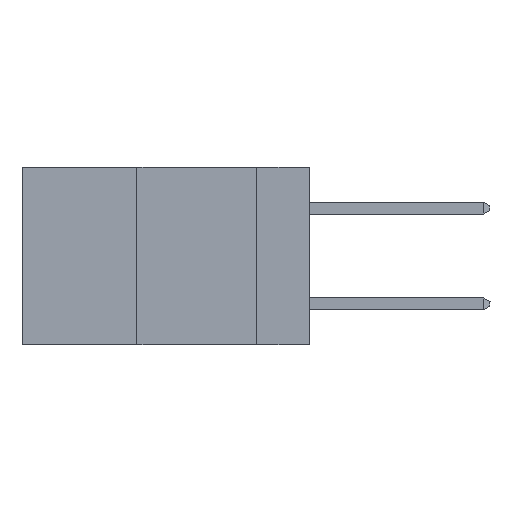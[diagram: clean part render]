
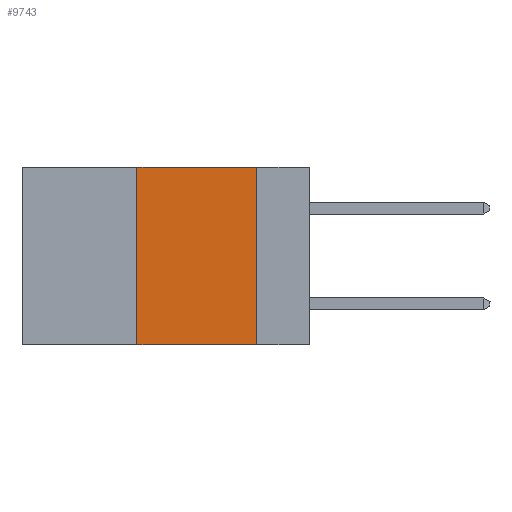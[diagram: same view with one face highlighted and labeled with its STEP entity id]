
A CAD part, left-side view. The second image highlights one B-rep face of the part: STEP entity #9743.
In plain terms, the highlighted planar face has unit normal (-1, 0, 0).
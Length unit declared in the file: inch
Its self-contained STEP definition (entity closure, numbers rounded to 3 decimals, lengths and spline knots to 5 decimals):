
#1336 = VERTEX_POINT ( 'NONE', #26502 ) ;
#2044 = CARTESIAN_POINT ( 'NONE',  ( 0., 0.11, 0. ) ) ;
#2357 = DIRECTION ( 'NONE',  ( 1., 0., 0. ) ) ;
#4958 = DIRECTION ( 'NONE',  ( 0., -1., 0. ) ) ;
#5106 = EDGE_CURVE ( 'NONE', #9497, #31726, #23253, .T. ) ;
#5832 = ORIENTED_EDGE ( 'NONE', *, *, #11111, .F. ) ;
#6289 = LINE ( 'NONE', #7561, #10682 ) ;
#7217 = VECTOR ( 'NONE', #33815, 39.37008 ) ;
#7561 = CARTESIAN_POINT ( 'NONE',  ( 0., 0.6, -0.37 ) ) ;
#7718 = CARTESIAN_POINT ( 'NONE',  ( 0., 0.36, 0. ) ) ;
#9497 = VERTEX_POINT ( 'NONE', #12365 ) ;
#9743 = ADVANCED_FACE ( 'NONE', ( #30087 ), #16248, .F. ) ;
#9936 = CARTESIAN_POINT ( 'NONE',  ( 0., 0.36, 0. ) ) ;
#10573 = EDGE_LOOP ( 'NONE', ( #14742, #5832, #19377, #34972 ) ) ;
#10581 = EDGE_CURVE ( 'NONE', #9497, #23884, #6289, .T. ) ;
#10682 = VECTOR ( 'NONE', #4958, 39.37008 ) ;
#10833 = CARTESIAN_POINT ( 'NONE',  ( 0., 0.6, 0. ) ) ;
#11111 = EDGE_CURVE ( 'NONE', #31726, #1336, #33546, .T. ) ;
#11413 = DIRECTION ( 'NONE',  ( 0., 0., -1. ) ) ;
#11894 = EDGE_CURVE ( 'NONE', #1336, #23884, #26454, .T. ) ;
#12365 = CARTESIAN_POINT ( 'NONE',  ( 0., 0.36, -0.37 ) ) ;
#12516 = CARTESIAN_POINT ( 'NONE',  ( 0., 0.11, -0.37 ) ) ;
#14742 = ORIENTED_EDGE ( 'NONE', *, *, #11894, .F. ) ;
#16248 = PLANE ( 'NONE',  #36211 ) ;
#18079 = VECTOR ( 'NONE', #11413, 39.37008 ) ;
#19377 = ORIENTED_EDGE ( 'NONE', *, *, #5106, .F. ) ;
#23253 = LINE ( 'NONE', #7718, #30719 ) ;
#23884 = VERTEX_POINT ( 'NONE', #12516 ) ;
#24943 = DIRECTION ( 'NONE',  ( 0., 0., -1. ) ) ;
#26454 = LINE ( 'NONE', #2044, #18079 ) ;
#26502 = CARTESIAN_POINT ( 'NONE',  ( 0., 0.11, 0. ) ) ;
#27431 = CARTESIAN_POINT ( 'NONE',  ( 0., 0.6, 0. ) ) ;
#29802 = DIRECTION ( 'NONE',  ( 0., 0., 1. ) ) ;
#30087 = FACE_OUTER_BOUND ( 'NONE', #10573, .T. ) ;
#30719 = VECTOR ( 'NONE', #29802, 39.37008 ) ;
#31726 = VERTEX_POINT ( 'NONE', #9936 ) ;
#33546 = LINE ( 'NONE', #10833, #7217 ) ;
#33815 = DIRECTION ( 'NONE',  ( 0., -1., 0. ) ) ;
#34972 = ORIENTED_EDGE ( 'NONE', *, *, #10581, .T. ) ;
#36211 = AXIS2_PLACEMENT_3D ( 'NONE', #27431, #2357, #24943 ) ;
